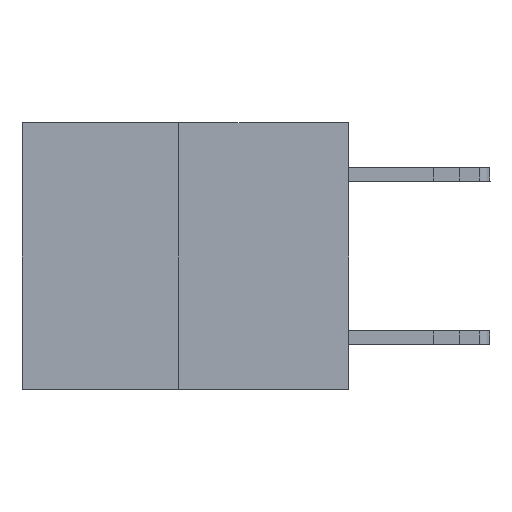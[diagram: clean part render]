
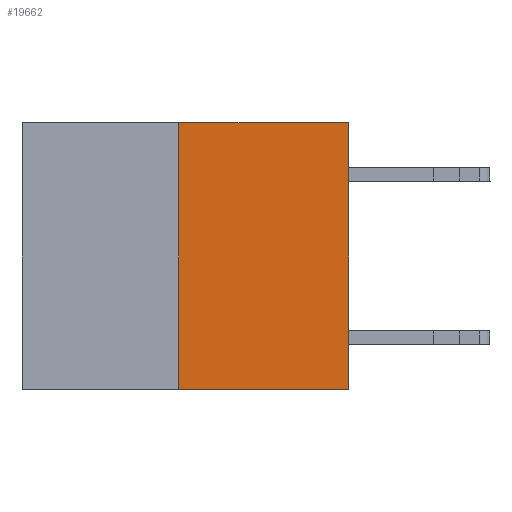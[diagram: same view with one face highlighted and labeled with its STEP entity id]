
A CAD part, left-side view. The second image highlights one B-rep face of the part: STEP entity #19662.
In plain terms, the highlighted planar face has unit normal (-1, 0, 0).
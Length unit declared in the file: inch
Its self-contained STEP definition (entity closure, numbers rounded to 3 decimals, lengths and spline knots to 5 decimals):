
#587 = VERTEX_POINT ( 'NONE', #7539 ) ;
#1123 = CARTESIAN_POINT ( 'NONE',  ( 0., 0.312, -0.49 ) ) ;
#1364 = DIRECTION ( 'NONE',  ( 1., 0., 0. ) ) ;
#1407 = EDGE_CURVE ( 'NONE', #13950, #587, #2440, .T. ) ;
#1605 = PLANE ( 'NONE',  #20960 ) ;
#1896 = DIRECTION ( 'NONE',  ( 0., 0., 1. ) ) ;
#2145 = CARTESIAN_POINT ( 'NONE',  ( 0., 0., -0.49 ) ) ;
#2440 = LINE ( 'NONE', #8652, #10888 ) ;
#3029 = DIRECTION ( 'NONE',  ( 0., -1., 0. ) ) ;
#3784 = VERTEX_POINT ( 'NONE', #2145 ) ;
#5867 = EDGE_LOOP ( 'NONE', ( #17790, #22355, #15444, #22795 ) ) ;
#7490 = CARTESIAN_POINT ( 'NONE',  ( 0., 0.6, -0.49 ) ) ;
#7539 = CARTESIAN_POINT ( 'NONE',  ( 0., 0., 0. ) ) ;
#8652 = CARTESIAN_POINT ( 'NONE',  ( 0., 0.6, 0. ) ) ;
#8872 = EDGE_CURVE ( 'NONE', #18634, #13950, #19492, .T. ) ;
#9052 = FACE_OUTER_BOUND ( 'NONE', #5867, .T. ) ;
#9133 = CARTESIAN_POINT ( 'NONE',  ( 0., 0., 0. ) ) ;
#10888 = VECTOR ( 'NONE', #3029, 39.37008 ) ;
#11551 = LINE ( 'NONE', #7490, #23744 ) ;
#12422 = CARTESIAN_POINT ( 'NONE',  ( 0., 0.312, 0. ) ) ;
#13950 = VERTEX_POINT ( 'NONE', #12422 ) ;
#14597 = VECTOR ( 'NONE', #1896, 39.37008 ) ;
#15173 = LINE ( 'NONE', #9133, #14597 ) ;
#15444 = ORIENTED_EDGE ( 'NONE', *, *, #22769, .T. ) ;
#16568 = CARTESIAN_POINT ( 'NONE',  ( 0., 0.6, 0. ) ) ;
#16578 = VECTOR ( 'NONE', #20205, 39.37008 ) ;
#16650 = DIRECTION ( 'NONE',  ( 0., -1., 0. ) ) ;
#17790 = ORIENTED_EDGE ( 'NONE', *, *, #8872, .F. ) ;
#18102 = DIRECTION ( 'NONE',  ( 0., 0., -1. ) ) ;
#18574 = CARTESIAN_POINT ( 'NONE',  ( 0., 0.312, -0.49 ) ) ;
#18634 = VERTEX_POINT ( 'NONE', #1123 ) ;
#19492 = LINE ( 'NONE', #18574, #16578 ) ;
#19662 = ADVANCED_FACE ( 'NONE', ( #9052 ), #1605, .F. ) ;
#20205 = DIRECTION ( 'NONE',  ( 0., 0., 1. ) ) ;
#20960 = AXIS2_PLACEMENT_3D ( 'NONE', #16568, #1364, #18102 ) ;
#22137 = EDGE_CURVE ( 'NONE', #18634, #3784, #11551, .T. ) ;
#22355 = ORIENTED_EDGE ( 'NONE', *, *, #22137, .T. ) ;
#22769 = EDGE_CURVE ( 'NONE', #3784, #587, #15173, .T. ) ;
#22795 = ORIENTED_EDGE ( 'NONE', *, *, #1407, .F. ) ;
#23744 = VECTOR ( 'NONE', #16650, 39.37008 ) ;
